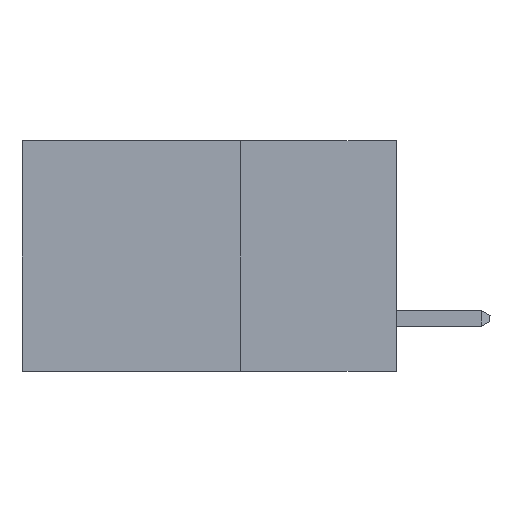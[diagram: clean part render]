
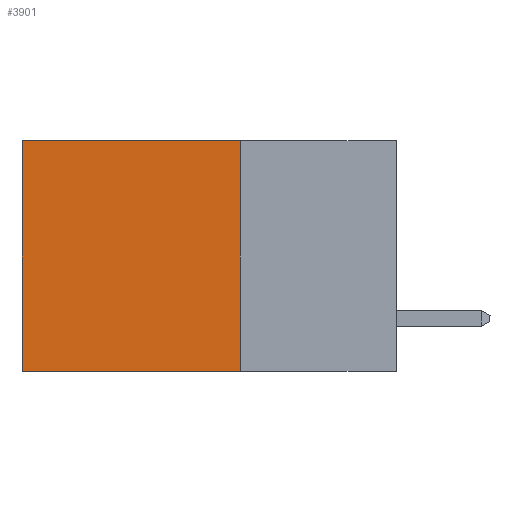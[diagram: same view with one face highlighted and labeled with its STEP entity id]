
A CAD part, left-side view. The second image highlights one B-rep face of the part: STEP entity #3901.
In plain terms, the highlighted planar face has unit normal (-1, 0, 0).
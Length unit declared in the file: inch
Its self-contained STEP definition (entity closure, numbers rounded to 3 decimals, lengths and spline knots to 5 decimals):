
#10 = DIRECTION ( 'NONE',  ( 0., 0., -1. ) ) ;
#120 = EDGE_LOOP ( 'NONE', ( #2563, #2584, #2726, #2747 ) ) ;
#615 = AXIS2_PLACEMENT_3D ( 'NONE', #8770, #8825, #10 ) ;
#1090 = CARTESIAN_POINT ( 'NONE',  ( 0.2615, 0.25, -0.37 ) ) ;
#1504 = VECTOR ( 'NONE', #5547, 39.37008 ) ;
#1761 = EDGE_CURVE ( 'NONE', #4704, #6944, #3918, .T. ) ;
#2170 = DIRECTION ( 'NONE',  ( 0., 0., -1. ) ) ;
#2426 = VECTOR ( 'NONE', #8987, 39.37008 ) ;
#2563 = ORIENTED_EDGE ( 'NONE', *, *, #7141, .T. ) ;
#2584 = ORIENTED_EDGE ( 'NONE', *, *, #4712, .F. ) ;
#2726 = ORIENTED_EDGE ( 'NONE', *, *, #10588, .F. ) ;
#2747 = ORIENTED_EDGE ( 'NONE', *, *, #1761, .T. ) ;
#3901 = ADVANCED_FACE ( 'NONE', ( #7016 ), #9262, .F. ) ;
#3918 = LINE ( 'NONE', #9613, #1504 ) ;
#4162 = VECTOR ( 'NONE', #2170, 39.37008 ) ;
#4439 = LINE ( 'NONE', #6750, #4162 ) ;
#4704 = VERTEX_POINT ( 'NONE', #10555 ) ;
#4712 = EDGE_CURVE ( 'NONE', #9939, #7361, #11235, .T. ) ;
#5547 = DIRECTION ( 'NONE',  ( 0., 1., 0. ) ) ;
#6127 = VECTOR ( 'NONE', #9114, 39.37008 ) ;
#6423 = LINE ( 'NONE', #9157, #6127 ) ;
#6750 = CARTESIAN_POINT ( 'NONE',  ( 0.2615, 0.25, -0.37 ) ) ;
#6944 = VERTEX_POINT ( 'NONE', #11204 ) ;
#7016 = FACE_OUTER_BOUND ( 'NONE', #120, .T. ) ;
#7141 = EDGE_CURVE ( 'NONE', #6944, #7361, #6423, .T. ) ;
#7361 = VERTEX_POINT ( 'NONE', #7559 ) ;
#7559 = CARTESIAN_POINT ( 'NONE',  ( 0.2615, 0.6, -0.37 ) ) ;
#8770 = CARTESIAN_POINT ( 'NONE',  ( 0.2615, 0.25, -0.37 ) ) ;
#8825 = DIRECTION ( 'NONE',  ( 1., 0., 0. ) ) ;
#8987 = DIRECTION ( 'NONE',  ( 0., 1., 0. ) ) ;
#9114 = DIRECTION ( 'NONE',  ( 0., 0., -1. ) ) ;
#9157 = CARTESIAN_POINT ( 'NONE',  ( 0.2615, 0.6, -0.37 ) ) ;
#9262 = PLANE ( 'NONE',  #615 ) ;
#9613 = CARTESIAN_POINT ( 'NONE',  ( 0.2615, 0.25, 0. ) ) ;
#9939 = VERTEX_POINT ( 'NONE', #1090 ) ;
#10300 = CARTESIAN_POINT ( 'NONE',  ( 0.2615, 0.25, -0.37 ) ) ;
#10555 = CARTESIAN_POINT ( 'NONE',  ( 0.2615, 0.25, 0. ) ) ;
#10588 = EDGE_CURVE ( 'NONE', #4704, #9939, #4439, .T. ) ;
#11204 = CARTESIAN_POINT ( 'NONE',  ( 0.2615, 0.6, 0. ) ) ;
#11235 = LINE ( 'NONE', #10300, #2426 ) ;
